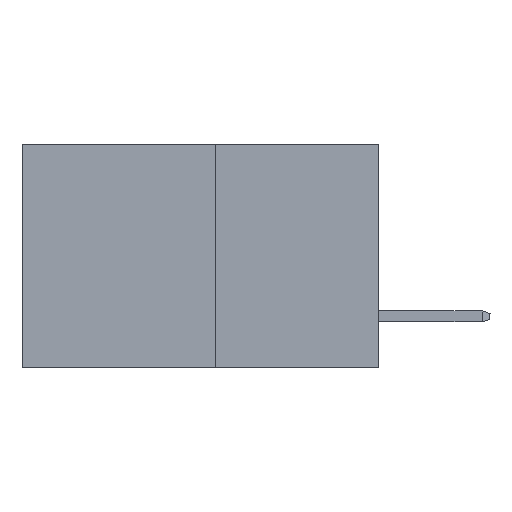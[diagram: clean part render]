
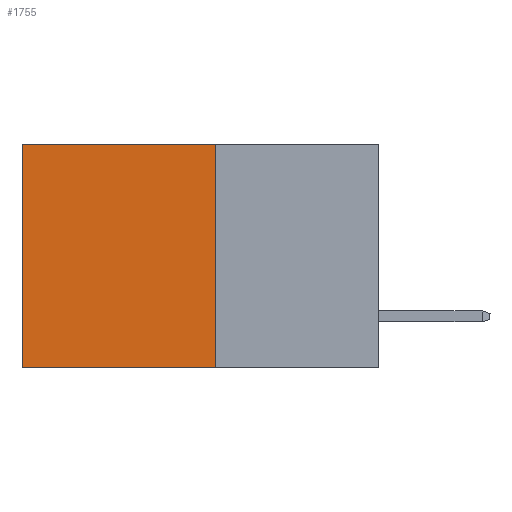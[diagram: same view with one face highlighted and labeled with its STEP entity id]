
A CAD part, left-side view. The second image highlights one B-rep face of the part: STEP entity #1755.
In plain terms, the highlighted planar face has unit normal (-1, 0, 0).
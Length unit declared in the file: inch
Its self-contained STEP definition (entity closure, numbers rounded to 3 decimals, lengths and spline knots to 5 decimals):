
#205 = EDGE_LOOP ( 'NONE', ( #2569, #1972, #8276, #9052 ) ) ;
#737 = CARTESIAN_POINT ( 'NONE',  ( 0.277, 0.27, 0. ) ) ;
#933 = CARTESIAN_POINT ( 'NONE',  ( 0.277, 0.27, 0. ) ) ;
#1198 = CARTESIAN_POINT ( 'NONE',  ( 0.277, 0.59, -0.37 ) ) ;
#1358 = CARTESIAN_POINT ( 'NONE',  ( 0.277, 0.27, -0.37 ) ) ;
#1443 = VECTOR ( 'NONE', #4430, 39.37008 ) ;
#1486 = DIRECTION ( 'NONE',  ( 0., 1., 0. ) ) ;
#1544 = DIRECTION ( 'NONE',  ( 0., 0., -1. ) ) ;
#1584 = VERTEX_POINT ( 'NONE', #933 ) ;
#1755 = ADVANCED_FACE ( 'NONE', ( #7200 ), #6665, .F. ) ;
#1882 = EDGE_CURVE ( 'NONE', #1584, #6049, #2122, .T. ) ;
#1950 = DIRECTION ( 'NONE',  ( 0., 0., -1. ) ) ;
#1972 = ORIENTED_EDGE ( 'NONE', *, *, #4291, .F. ) ;
#2122 = LINE ( 'NONE', #4885, #4138 ) ;
#2569 = ORIENTED_EDGE ( 'NONE', *, *, #7798, .T. ) ;
#2695 = CARTESIAN_POINT ( 'NONE',  ( 0.277, 0.59, 0. ) ) ;
#2812 = CARTESIAN_POINT ( 'NONE',  ( 0.277, 0.27, -0.37 ) ) ;
#3147 = DIRECTION ( 'NONE',  ( 0., 0., -1. ) ) ;
#4138 = VECTOR ( 'NONE', #1544, 39.37008 ) ;
#4291 = EDGE_CURVE ( 'NONE', #6049, #7848, #7322, .T. ) ;
#4430 = DIRECTION ( 'NONE',  ( 0., 1., 0. ) ) ;
#4497 = AXIS2_PLACEMENT_3D ( 'NONE', #2812, #9168, #3147 ) ;
#4885 = CARTESIAN_POINT ( 'NONE',  ( 0.277, 0.27, -0.37 ) ) ;
#5103 = VECTOR ( 'NONE', #1486, 39.37008 ) ;
#6049 = VERTEX_POINT ( 'NONE', #1358 ) ;
#6665 = PLANE ( 'NONE',  #4497 ) ;
#7051 = VECTOR ( 'NONE', #1950, 39.37008 ) ;
#7200 = FACE_OUTER_BOUND ( 'NONE', #205, .T. ) ;
#7322 = LINE ( 'NONE', #8035, #1443 ) ;
#7798 = EDGE_CURVE ( 'NONE', #7822, #7848, #8947, .T. ) ;
#7822 = VERTEX_POINT ( 'NONE', #2695 ) ;
#7848 = VERTEX_POINT ( 'NONE', #8574 ) ;
#8035 = CARTESIAN_POINT ( 'NONE',  ( 0.277, 0.27, -0.37 ) ) ;
#8276 = ORIENTED_EDGE ( 'NONE', *, *, #1882, .F. ) ;
#8574 = CARTESIAN_POINT ( 'NONE',  ( 0.277, 0.59, -0.37 ) ) ;
#8931 = LINE ( 'NONE', #737, #5103 ) ;
#8947 = LINE ( 'NONE', #1198, #7051 ) ;
#9052 = ORIENTED_EDGE ( 'NONE', *, *, #9294, .T. ) ;
#9168 = DIRECTION ( 'NONE',  ( 1., 0., 0. ) ) ;
#9294 = EDGE_CURVE ( 'NONE', #1584, #7822, #8931, .T. ) ;
